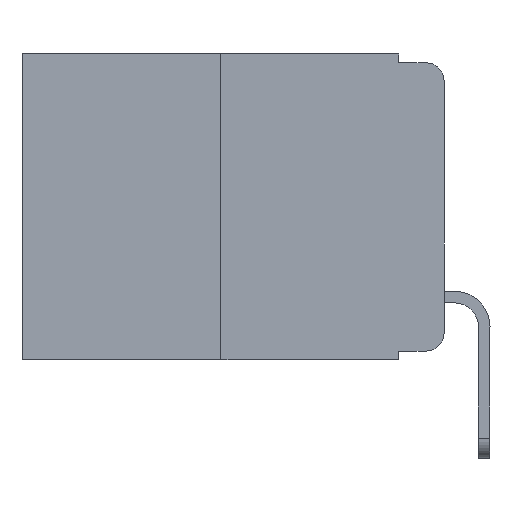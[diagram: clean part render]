
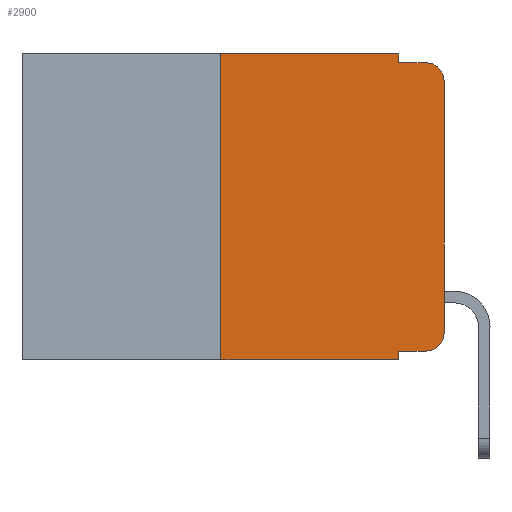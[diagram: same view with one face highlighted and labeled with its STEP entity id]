
A CAD part, left-side view. The second image highlights one B-rep face of the part: STEP entity #2900.
In plain terms, the highlighted planar face has unit normal (-1, 0, 0).
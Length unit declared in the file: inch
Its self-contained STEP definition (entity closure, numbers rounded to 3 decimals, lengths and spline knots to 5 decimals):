
#1033 = VECTOR ( 'NONE', #4764, 39.37008 ) ;
#1222 = AXIS2_PLACEMENT_3D ( 'NONE', #10142, #9972, #7871 ) ;
#1542 = CIRCLE ( 'NONE', #7805, 0.02 ) ;
#1612 = ORIENTED_EDGE ( 'NONE', *, *, #6633, .T. ) ;
#1615 = VERTEX_POINT ( 'NONE', #11694 ) ;
#1668 = DIRECTION ( 'NONE',  ( 0., -1., 0. ) ) ;
#1870 = DIRECTION ( 'NONE',  ( -1., 0., 0. ) ) ;
#2068 = LINE ( 'NONE', #3275, #11525 ) ;
#2157 = DIRECTION ( 'NONE',  ( 0., 0., -1. ) ) ;
#2272 = CARTESIAN_POINT ( 'NONE',  ( 0., 0.051, 0. ) ) ;
#2300 = EDGE_CURVE ( 'NONE', #3998, #3749, #8487, .T. ) ;
#2319 = VECTOR ( 'NONE', #7603, 39.37008 ) ;
#2336 = EDGE_CURVE ( 'NONE', #7215, #3998, #5666, .T. ) ;
#2432 = EDGE_CURVE ( 'NONE', #4809, #3342, #7055, .T. ) ;
#2519 = EDGE_CURVE ( 'NONE', #4991, #10898, #10957, .T. ) ;
#2882 = ORIENTED_EDGE ( 'NONE', *, *, #2300, .T. ) ;
#2900 = ADVANCED_FACE ( 'NONE', ( #6134 ), #5753, .F. ) ;
#3242 = CARTESIAN_POINT ( 'NONE',  ( 0., 0.02, -0.01 ) ) ;
#3275 = CARTESIAN_POINT ( 'NONE',  ( 0., 0., 0. ) ) ;
#3342 = VERTEX_POINT ( 'NONE', #5801 ) ;
#3440 = ORIENTED_EDGE ( 'NONE', *, *, #3742, .F. ) ;
#3482 = ORIENTED_EDGE ( 'NONE', *, *, #3890, .T. ) ;
#3685 = DIRECTION ( 'NONE',  ( 0., 0., 1. ) ) ;
#3742 = EDGE_CURVE ( 'NONE', #10898, #7414, #12392, .T. ) ;
#3749 = VERTEX_POINT ( 'NONE', #9361 ) ;
#3890 = EDGE_CURVE ( 'NONE', #4809, #8249, #9388, .T. ) ;
#3957 = ORIENTED_EDGE ( 'NONE', *, *, #2336, .T. ) ;
#3998 = VERTEX_POINT ( 'NONE', #4259 ) ;
#4042 = ORIENTED_EDGE ( 'NONE', *, *, #2432, .F. ) ;
#4259 = CARTESIAN_POINT ( 'NONE',  ( 0., 0.02, -0.333 ) ) ;
#4364 = ORIENTED_EDGE ( 'NONE', *, *, #7211, .T. ) ;
#4444 = CARTESIAN_POINT ( 'NONE',  ( 0., 0.051, -0.333 ) ) ;
#4664 = VECTOR ( 'NONE', #1668, 39.37008 ) ;
#4764 = DIRECTION ( 'NONE',  ( 0., 0., -1. ) ) ;
#4809 = VERTEX_POINT ( 'NONE', #10996 ) ;
#4991 = VERTEX_POINT ( 'NONE', #2272 ) ;
#5242 = CARTESIAN_POINT ( 'NONE',  ( 0., 0.473, -0.343 ) ) ;
#5274 = DIRECTION ( 'NONE',  ( 0., 0., -1. ) ) ;
#5487 = ORIENTED_EDGE ( 'NONE', *, *, #7475, .F. ) ;
#5666 = LINE ( 'NONE', #10528, #8232 ) ;
#5753 = PLANE ( 'NONE',  #7899 ) ;
#5801 = CARTESIAN_POINT ( 'NONE',  ( 0., 0.25, 0. ) ) ;
#5846 = CARTESIAN_POINT ( 'NONE',  ( 0., 0.051, 0. ) ) ;
#6134 = FACE_OUTER_BOUND ( 'NONE', #10246, .T. ) ;
#6182 = LINE ( 'NONE', #5846, #1033 ) ;
#6303 = DIRECTION ( 'NONE',  ( 0., 0., -1. ) ) ;
#6416 = DIRECTION ( 'NONE',  ( 1., 0., 0. ) ) ;
#6469 = VECTOR ( 'NONE', #8189, 39.37008 ) ;
#6606 = CARTESIAN_POINT ( 'NONE',  ( 0., 0.25, 0. ) ) ;
#6633 = EDGE_CURVE ( 'NONE', #3749, #1615, #2068, .T. ) ;
#7055 = LINE ( 'NONE', #6606, #2319 ) ;
#7175 = ORIENTED_EDGE ( 'NONE', *, *, #7452, .F. ) ;
#7211 = EDGE_CURVE ( 'NONE', #1615, #7414, #1542, .T. ) ;
#7215 = VERTEX_POINT ( 'NONE', #4444 ) ;
#7414 = VERTEX_POINT ( 'NONE', #3242 ) ;
#7452 = EDGE_CURVE ( 'NONE', #3342, #4991, #9198, .T. ) ;
#7475 = EDGE_CURVE ( 'NONE', #7215, #8249, #6182, .T. ) ;
#7481 = ORIENTED_EDGE ( 'NONE', *, *, #2519, .F. ) ;
#7603 = DIRECTION ( 'NONE',  ( 0., 0., 1. ) ) ;
#7805 = AXIS2_PLACEMENT_3D ( 'NONE', #10571, #1870, #2157 ) ;
#7871 = DIRECTION ( 'NONE',  ( 0., 0., -1. ) ) ;
#7899 = AXIS2_PLACEMENT_3D ( 'NONE', #11751, #6416, #5274 ) ;
#8085 = CARTESIAN_POINT ( 'NONE',  ( 0., 0.051, -0.01 ) ) ;
#8189 = DIRECTION ( 'NONE',  ( 0., -1., 0. ) ) ;
#8232 = VECTOR ( 'NONE', #9521, 39.37008 ) ;
#8249 = VERTEX_POINT ( 'NONE', #8596 ) ;
#8355 = VECTOR ( 'NONE', #6303, 39.37008 ) ;
#8487 = CIRCLE ( 'NONE', #1222, 0.02 ) ;
#8522 = CARTESIAN_POINT ( 'NONE',  ( 0., 0.051, -0.01 ) ) ;
#8596 = CARTESIAN_POINT ( 'NONE',  ( 0., 0.051, -0.343 ) ) ;
#9198 = LINE ( 'NONE', #11856, #6469 ) ;
#9361 = CARTESIAN_POINT ( 'NONE',  ( 0., 0., -0.313 ) ) ;
#9388 = LINE ( 'NONE', #5242, #4664 ) ;
#9508 = CARTESIAN_POINT ( 'NONE',  ( 0., 0.051, 0. ) ) ;
#9521 = DIRECTION ( 'NONE',  ( 0., -1., 0. ) ) ;
#9738 = DIRECTION ( 'NONE',  ( 0., -1., 0. ) ) ;
#9972 = DIRECTION ( 'NONE',  ( -1., 0., 0. ) ) ;
#10142 = CARTESIAN_POINT ( 'NONE',  ( 0., 0.02, -0.313 ) ) ;
#10246 = EDGE_LOOP ( 'NONE', ( #1612, #4364, #3440, #7481, #7175, #4042, #3482, #5487, #3957, #2882 ) ) ;
#10528 = CARTESIAN_POINT ( 'NONE',  ( 0., 0.051, -0.333 ) ) ;
#10571 = CARTESIAN_POINT ( 'NONE',  ( 0., 0.02, -0.03 ) ) ;
#10898 = VERTEX_POINT ( 'NONE', #8522 ) ;
#10957 = LINE ( 'NONE', #9508, #8355 ) ;
#10996 = CARTESIAN_POINT ( 'NONE',  ( 0., 0.25, -0.343 ) ) ;
#11525 = VECTOR ( 'NONE', #3685, 39.37008 ) ;
#11694 = CARTESIAN_POINT ( 'NONE',  ( 0., 0., -0.03 ) ) ;
#11751 = CARTESIAN_POINT ( 'NONE',  ( 0., 0.473, 0. ) ) ;
#11856 = CARTESIAN_POINT ( 'NONE',  ( 0., 0.473, 0. ) ) ;
#12104 = VECTOR ( 'NONE', #9738, 39.37008 ) ;
#12392 = LINE ( 'NONE', #8085, #12104 ) ;
